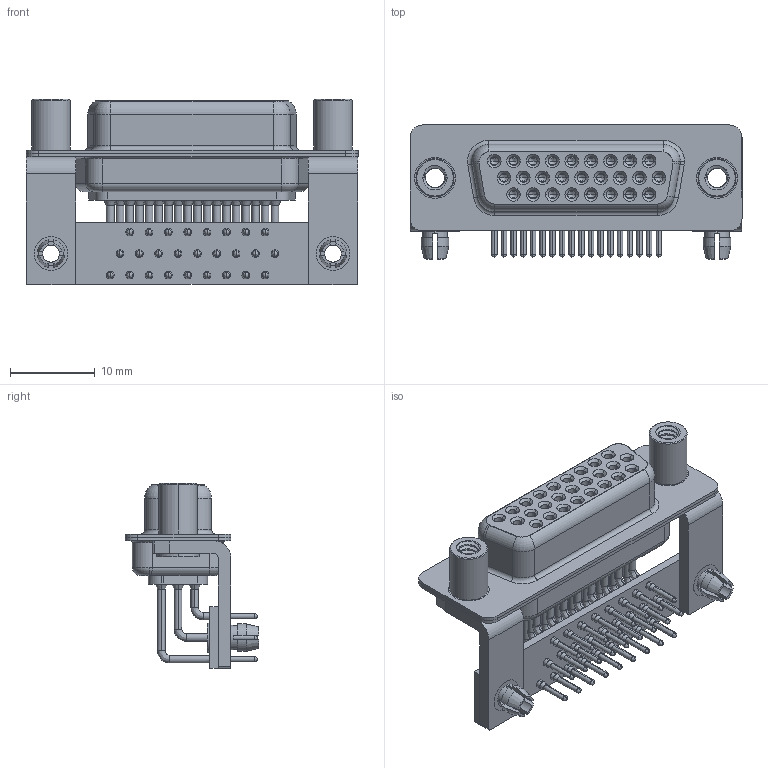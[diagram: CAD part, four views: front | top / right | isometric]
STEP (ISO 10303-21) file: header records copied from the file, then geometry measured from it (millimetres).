
FILE_DESCRIPTION (( 'STEP AP203' ), '1' );
FILE_NAME ('634-M26-263-BT5.STEP', '2018-09-27T22:40:06', ( '' ), ( '' ), 'SwSTEP 2.0', 'SolidWorks 2016', '' );
FILE_SCHEMA (( 'CONFIG_CONTROL_DESIGN' ));
Length unit declared in the file: millimetre
Products named in the file (11): 634-M26-263-BT5; 634M Contact Row 1; 634M Contact Row 2; 634M Contact Row 3; 634M Stabilizer Bracket; 634M Housing_26 Contacts; 634M 4-40 Threaded Standoff; 634M Shell Front_26 Contacts; 634M Stabilizer Board_26 Contacts; 634M Shell Rear_26 Contacts; 634M Board Lock
Assembly tree (36 placements, depth 2):
  634-M26-263-BT5
    634M Housing_26 Contacts
    634M Shell Front_26 Contacts
    634M Shell Rear_26 Contacts
    634M Contact Row 1  x9
    634M Contact Row 2  x9
    634M Contact Row 3  x8
    634M Stabilizer Bracket  x2
    634M 4-40 Threaded Standoff  x2
    634M Stabilizer Board_26 Contacts
    634M Board Lock  x2
Bounding box: 39.2 x 15.8 x 21.9 mm (x, y, z)
Volume: 3236.3 mm3; surface area: 10333.3 mm2
Topology: 36 solids, 36 shells, 1901 faces, 4865 edges, 3079 vertices
Faces by surface type: cylinder 883, plane 533, cone 312, bspline 110, torus 63
Entity records: 29552 total; most frequent: CARTESIAN_POINT 6665, DIRECTION 4789, ORIENTED_EDGE 4132, EDGE_CURVE 2066, AXIS2_PLACEMENT_3D 1985, VERTEX_POINT 1325, CIRCLE 1104, EDGE_LOOP 1081
